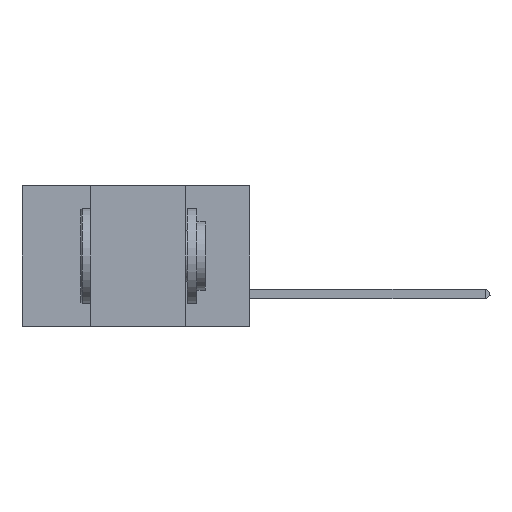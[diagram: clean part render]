
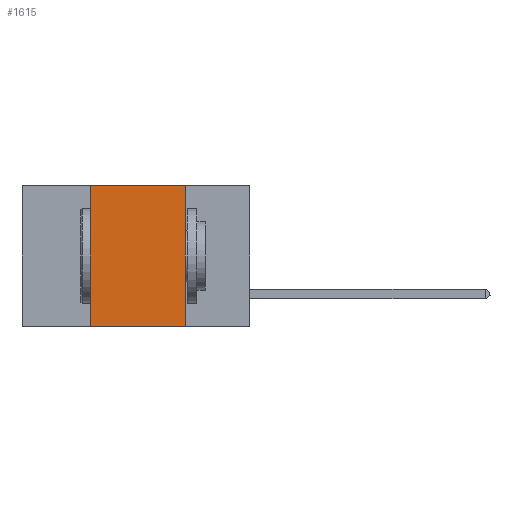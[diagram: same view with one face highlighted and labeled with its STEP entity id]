
A CAD part, left-side view. The second image highlights one B-rep face of the part: STEP entity #1615.
In plain terms, the highlighted planar face has unit normal (-1, 0, 0).
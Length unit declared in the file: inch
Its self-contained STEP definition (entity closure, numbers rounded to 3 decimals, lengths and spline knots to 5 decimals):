
#233 = CARTESIAN_POINT ( 'NONE',  ( 0., 0.17, 0. ) ) ;
#660 = VECTOR ( 'NONE', #14057, 39.37008 ) ;
#1479 = DIRECTION ( 'NONE',  ( 0., 0., 1. ) ) ;
#1615 = ADVANCED_FACE ( 'NONE', ( #21258 ), #10543, .F. ) ;
#2361 = EDGE_CURVE ( 'NONE', #17544, #6655, #21211, .T. ) ;
#4101 = EDGE_CURVE ( 'NONE', #23638, #6655, #23858, .T. ) ;
#4350 = CARTESIAN_POINT ( 'NONE',  ( 0., 0.42, 0. ) ) ;
#4707 = CARTESIAN_POINT ( 'NONE',  ( 0., 0.42, 0. ) ) ;
#4991 = AXIS2_PLACEMENT_3D ( 'NONE', #8421, #10645, #21259 ) ;
#6134 = CARTESIAN_POINT ( 'NONE',  ( 0., 0.17, -0.37 ) ) ;
#6655 = VERTEX_POINT ( 'NONE', #6134 ) ;
#6847 = EDGE_LOOP ( 'NONE', ( #20581, #15831, #6982, #12836 ) ) ;
#6982 = ORIENTED_EDGE ( 'NONE', *, *, #9934, .F. ) ;
#7142 = CARTESIAN_POINT ( 'NONE',  ( 0., 0.17, 0. ) ) ;
#8394 = VECTOR ( 'NONE', #1479, 39.37008 ) ;
#8421 = CARTESIAN_POINT ( 'NONE',  ( 0., 0.6, 0. ) ) ;
#9934 = EDGE_CURVE ( 'NONE', #17544, #27815, #22562, .T. ) ;
#10543 = PLANE ( 'NONE',  #4991 ) ;
#10645 = DIRECTION ( 'NONE',  ( 1., 0., 0. ) ) ;
#11426 = EDGE_CURVE ( 'NONE', #27815, #23638, #27658, .T. ) ;
#12836 = ORIENTED_EDGE ( 'NONE', *, *, #2361, .T. ) ;
#14057 = DIRECTION ( 'NONE',  ( 0., 0., -1. ) ) ;
#15111 = CARTESIAN_POINT ( 'NONE',  ( 0., 0.6, 0. ) ) ;
#15831 = ORIENTED_EDGE ( 'NONE', *, *, #11426, .F. ) ;
#17544 = VERTEX_POINT ( 'NONE', #22445 ) ;
#20513 = VECTOR ( 'NONE', #20677, 39.37008 ) ;
#20581 = ORIENTED_EDGE ( 'NONE', *, *, #4101, .F. ) ;
#20677 = DIRECTION ( 'NONE',  ( 0., -1., 0. ) ) ;
#21211 = LINE ( 'NONE', #27219, #20513 ) ;
#21258 = FACE_OUTER_BOUND ( 'NONE', #6847, .T. ) ;
#21259 = DIRECTION ( 'NONE',  ( 0., 0., -1. ) ) ;
#22445 = CARTESIAN_POINT ( 'NONE',  ( 0., 0.42, -0.37 ) ) ;
#22562 = LINE ( 'NONE', #4350, #8394 ) ;
#23514 = VECTOR ( 'NONE', #24318, 39.37008 ) ;
#23638 = VERTEX_POINT ( 'NONE', #7142 ) ;
#23858 = LINE ( 'NONE', #233, #660 ) ;
#24318 = DIRECTION ( 'NONE',  ( 0., -1., 0. ) ) ;
#27219 = CARTESIAN_POINT ( 'NONE',  ( 0., 0.6, -0.37 ) ) ;
#27658 = LINE ( 'NONE', #15111, #23514 ) ;
#27815 = VERTEX_POINT ( 'NONE', #4707 ) ;
